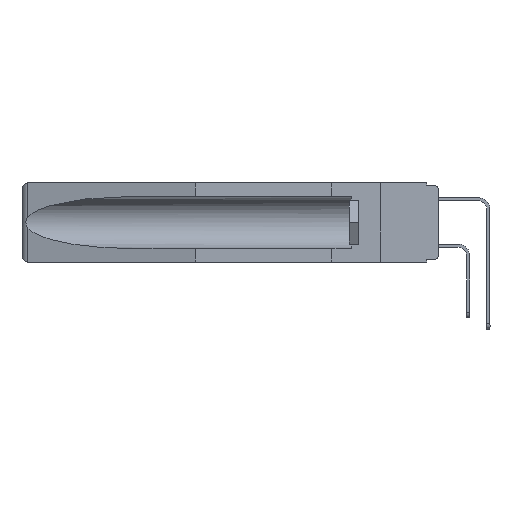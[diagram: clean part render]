
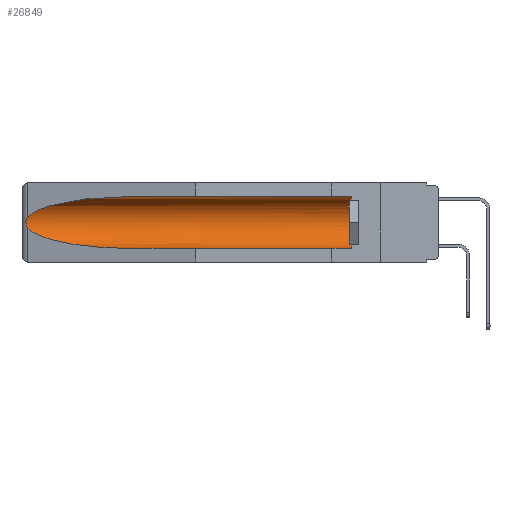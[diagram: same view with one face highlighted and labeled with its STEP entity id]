
A CAD part, left-side view. The second image highlights one B-rep face of the part: STEP entity #26849.
In plain terms, the highlighted cylindrical face has radius 2.857 mm (diameter 5.715 mm), a partial arc.
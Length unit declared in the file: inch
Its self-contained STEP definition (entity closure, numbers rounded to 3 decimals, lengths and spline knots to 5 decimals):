
#532 =( BOUNDED_CURVE ( )  B_SPLINE_CURVE ( 3, ( #15126, #4548, #13171, #13025 ),
 .UNSPECIFIED., .F., .F. ) 
 B_SPLINE_CURVE_WITH_KNOTS ( ( 4, 4 ),
 ( 4.71239, 6.08839 ),
 .UNSPECIFIED. ) 
 CURVE ( )  GEOMETRIC_REPRESENTATION_ITEM ( )  RATIONAL_B_SPLINE_CURVE ( ( 1., 0.848, 0.848, 1. ) ) 
 REPRESENTATION_ITEM ( '' )  );
#1176 = CARTESIAN_POINT ( 'NONE',  ( 0.155, -0.30754, -0.1715 ) ) ;
#2381 = AXIS2_PLACEMENT_3D ( 'NONE', #9313, #7509, #7098 ) ;
#2863 = CARTESIAN_POINT ( 'NONE',  ( 0.26597, 1.52961, -0.15275 ) ) ;
#3103 = VERTEX_POINT ( 'NONE', #17552 ) ;
#3302 = LINE ( 'NONE', #15965, #25046 ) ;
#3378 =( BOUNDED_CURVE ( )  B_SPLINE_CURVE ( 3, ( #11366, #19862, #23773, #24177 ),
 .UNSPECIFIED., .F., .F. ) 
 B_SPLINE_CURVE_WITH_KNOTS ( ( 4, 4 ),
 ( 0.1948, 1.5708 ),
 .UNSPECIFIED. ) 
 CURVE ( )  GEOMETRIC_REPRESENTATION_ITEM ( )  RATIONAL_B_SPLINE_CURVE ( ( 1., 0.848, 0.848, 1. ) ) 
 REPRESENTATION_ITEM ( '' )  );
#3541 = CYLINDRICAL_SURFACE ( 'NONE', #22617, 0.1125 ) ;
#4548 = CARTESIAN_POINT ( 'NONE',  ( 0.21114, 1.30732, -0.059 ) ) ;
#5491 = CARTESIAN_POINT ( 'NONE',  ( 0.26597, 1.5296, -0.19026 ) ) ;
#5608 = ORIENTED_EDGE ( 'NONE', *, *, #19140, .T. ) ;
#5881 = CARTESIAN_POINT ( 'NONE',  ( 0.26537, 1.52718, -0.14972 ) ) ;
#5902 = DIRECTION ( 'NONE',  ( 0., 1., 0. ) ) ;
#6332 = ORIENTED_EDGE ( 'NONE', *, *, #7418, .F. ) ;
#7098 = DIRECTION ( 'NONE',  ( 0., 0., 1. ) ) ;
#7124 = VERTEX_POINT ( 'NONE', #19558 ) ;
#7177 = CARTESIAN_POINT ( 'NONE',  ( 0.26654, 1.53092, -0.15636 ) ) ;
#7418 = EDGE_CURVE ( 'NONE', #3103, #19969, #14838, .T. ) ;
#7509 = DIRECTION ( 'NONE',  ( 0., -1., 0. ) ) ;
#8896 = ORIENTED_EDGE ( 'NONE', *, *, #15962, .T. ) ;
#9313 = CARTESIAN_POINT ( 'NONE',  ( 0.155, 0.126, -0.1715 ) ) ;
#9452 = CARTESIAN_POINT ( 'NONE',  ( 0.26537, 1.52718, -0.19328 ) ) ;
#9554 = DIRECTION ( 'NONE',  ( 0., 1., 0. ) ) ;
#9649 = VERTEX_POINT ( 'NONE', #5881 ) ;
#9725 = VECTOR ( 'NONE', #10383, 39.37008 ) ;
#10065 = CARTESIAN_POINT ( 'NONE',  ( 0.26655, 1.53094, -0.18657 ) ) ;
#10383 = DIRECTION ( 'NONE',  ( 0., 1., 0. ) ) ;
#10990 = B_SPLINE_CURVE_WITH_KNOTS ( 'NONE', 3,
 ( #26236, #2863, #7177, #11330, #19825, #13968, #22462, #10065, #5491, #12142 ),
 .UNSPECIFIED., .F., .F.,
 ( 4, 2, 2, 2, 4 ),
 ( 0., 0.00029, 0.00058, 0.00087, 0.00117 ),
 .UNSPECIFIED. ) ;
#11330 = CARTESIAN_POINT ( 'NONE',  ( 0.2673, 1.5327, -0.16383 ) ) ;
#11366 = CARTESIAN_POINT ( 'NONE',  ( 0.26537, 1.52718, -0.19328 ) ) ;
#11774 = ORIENTED_EDGE ( 'NONE', *, *, #21812, .T. ) ;
#12014 = DIRECTION ( 'NONE',  ( 0., 0., 1. ) ) ;
#12142 = CARTESIAN_POINT ( 'NONE',  ( 0.26537, 1.52718, -0.19328 ) ) ;
#13025 = CARTESIAN_POINT ( 'NONE',  ( 0.26537, 1.52718, -0.14972 ) ) ;
#13046 = ORIENTED_EDGE ( 'NONE', *, *, #26730, .T. ) ;
#13171 = CARTESIAN_POINT ( 'NONE',  ( 0.25451, 1.48313, -0.09465 ) ) ;
#13968 = CARTESIAN_POINT ( 'NONE',  ( 0.2675, 1.53308, -0.17534 ) ) ;
#14838 = LINE ( 'NONE', #23331, #9725 ) ;
#15126 = CARTESIAN_POINT ( 'NONE',  ( 0.155, 1.07973, -0.059 ) ) ;
#15962 = EDGE_CURVE ( 'NONE', #22380, #9649, #532, .T. ) ;
#15965 = CARTESIAN_POINT ( 'NONE',  ( 0.155, -0.30754, -0.059 ) ) ;
#16520 = ORIENTED_EDGE ( 'NONE', *, *, #17319, .T. ) ;
#17319 = EDGE_CURVE ( 'NONE', #7124, #22380, #3302, .T. ) ;
#17552 = CARTESIAN_POINT ( 'NONE',  ( 0.155, 0.126, -0.284 ) ) ;
#19140 = EDGE_CURVE ( 'NONE', #21834, #19969, #3378, .T. ) ;
#19558 = CARTESIAN_POINT ( 'NONE',  ( 0.155, 0.126, -0.059 ) ) ;
#19759 = CARTESIAN_POINT ( 'NONE',  ( 0.155, 1.07973, -0.284 ) ) ;
#19825 = CARTESIAN_POINT ( 'NONE',  ( 0.2675, 1.53308, -0.16763 ) ) ;
#19862 = CARTESIAN_POINT ( 'NONE',  ( 0.25451, 1.48313, -0.24835 ) ) ;
#19969 = VERTEX_POINT ( 'NONE', #19759 ) ;
#20240 = FACE_OUTER_BOUND ( 'NONE', #25117, .T. ) ;
#21812 = EDGE_CURVE ( 'NONE', #3103, #7124, #27270, .T. ) ;
#21834 = VERTEX_POINT ( 'NONE', #9452 ) ;
#22380 = VERTEX_POINT ( 'NONE', #22893 ) ;
#22462 = CARTESIAN_POINT ( 'NONE',  ( 0.2673, 1.53269, -0.17917 ) ) ;
#22617 = AXIS2_PLACEMENT_3D ( 'NONE', #1176, #5902, #12014 ) ;
#22893 = CARTESIAN_POINT ( 'NONE',  ( 0.155, 1.07973, -0.059 ) ) ;
#23331 = CARTESIAN_POINT ( 'NONE',  ( 0.155, -0.30754, -0.284 ) ) ;
#23773 = CARTESIAN_POINT ( 'NONE',  ( 0.21114, 1.30732, -0.284 ) ) ;
#24177 = CARTESIAN_POINT ( 'NONE',  ( 0.155, 1.07973, -0.284 ) ) ;
#25046 = VECTOR ( 'NONE', #9554, 39.37008 ) ;
#25117 = EDGE_LOOP ( 'NONE', ( #8896, #13046, #5608, #6332, #11774, #16520 ) ) ;
#26236 = CARTESIAN_POINT ( 'NONE',  ( 0.26537, 1.52718, -0.14972 ) ) ;
#26730 = EDGE_CURVE ( 'NONE', #9649, #21834, #10990, .T. ) ;
#26849 = ADVANCED_FACE ( 'NONE', ( #20240 ), #3541, .F. ) ;
#27270 = CIRCLE ( 'NONE', #2381, 0.1125 ) ;
